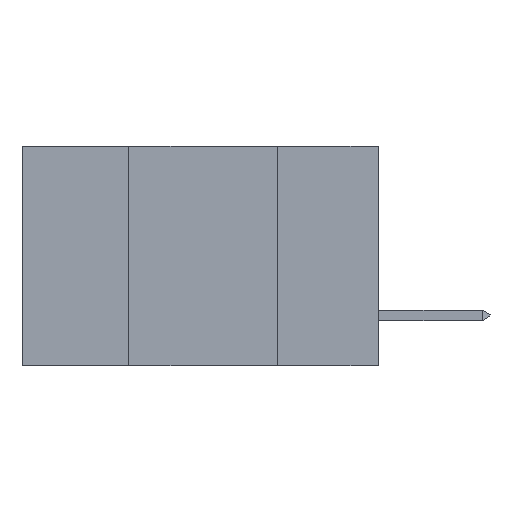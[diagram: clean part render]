
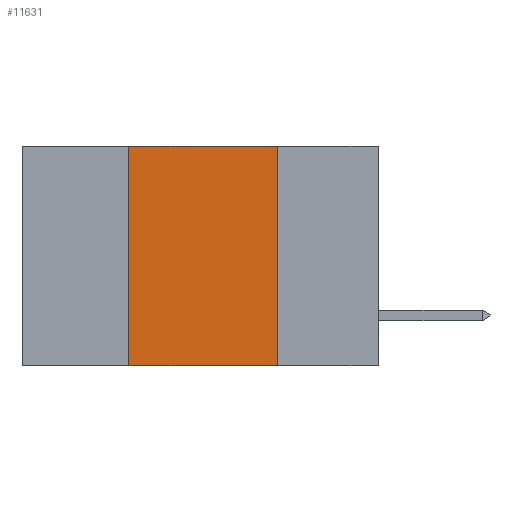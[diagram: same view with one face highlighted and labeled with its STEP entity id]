
A CAD part, left-side view. The second image highlights one B-rep face of the part: STEP entity #11631.
In plain terms, the highlighted planar face has unit normal (-1, 0, 0).
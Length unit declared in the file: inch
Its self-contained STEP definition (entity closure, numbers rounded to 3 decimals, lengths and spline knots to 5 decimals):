
#169 = DIRECTION ( 'NONE',  ( 0., -1., 0. ) ) ;
#295 = FACE_OUTER_BOUND ( 'NONE', #2165, .T. ) ;
#682 = CARTESIAN_POINT ( 'NONE',  ( 0., 0.17, -0.37 ) ) ;
#980 = LINE ( 'NONE', #7083, #4422 ) ;
#1053 = DIRECTION ( 'NONE',  ( 0., 0., -1. ) ) ;
#1113 = ORIENTED_EDGE ( 'NONE', *, *, #5870, .F. ) ;
#1149 = VERTEX_POINT ( 'NONE', #6041 ) ;
#1762 = EDGE_CURVE ( 'NONE', #8543, #9903, #980, .T. ) ;
#2165 = EDGE_LOOP ( 'NONE', ( #9676, #13576, #1113, #6295 ) ) ;
#2291 = LINE ( 'NONE', #9536, #14117 ) ;
#2891 = DIRECTION ( 'NONE',  ( 0., 0., -1. ) ) ;
#3404 = CARTESIAN_POINT ( 'NONE',  ( 0., 0.6, 0. ) ) ;
#3687 = DIRECTION ( 'NONE',  ( 0., -1., 0. ) ) ;
#4422 = VECTOR ( 'NONE', #169, 39.37008 ) ;
#5262 = CARTESIAN_POINT ( 'NONE',  ( 0., 0.42, -0.37 ) ) ;
#5268 = VERTEX_POINT ( 'NONE', #5733 ) ;
#5733 = CARTESIAN_POINT ( 'NONE',  ( 0., 0.42, 0. ) ) ;
#5734 = VECTOR ( 'NONE', #13889, 39.37008 ) ;
#5870 = EDGE_CURVE ( 'NONE', #8543, #5268, #11938, .T. ) ;
#6041 = CARTESIAN_POINT ( 'NONE',  ( 0., 0.17, 0. ) ) ;
#6295 = ORIENTED_EDGE ( 'NONE', *, *, #1762, .T. ) ;
#6999 = CARTESIAN_POINT ( 'NONE',  ( 0., 0.6, 0. ) ) ;
#7083 = CARTESIAN_POINT ( 'NONE',  ( 0., 0.6, -0.37 ) ) ;
#8543 = VERTEX_POINT ( 'NONE', #5262 ) ;
#8721 = AXIS2_PLACEMENT_3D ( 'NONE', #3404, #10389, #1053 ) ;
#8951 = VECTOR ( 'NONE', #3687, 39.37008 ) ;
#8956 = EDGE_CURVE ( 'NONE', #1149, #9903, #2291, .T. ) ;
#9357 = CARTESIAN_POINT ( 'NONE',  ( 0., 0.42, 0. ) ) ;
#9536 = CARTESIAN_POINT ( 'NONE',  ( 0., 0.17, 0. ) ) ;
#9676 = ORIENTED_EDGE ( 'NONE', *, *, #8956, .F. ) ;
#9903 = VERTEX_POINT ( 'NONE', #682 ) ;
#10246 = PLANE ( 'NONE',  #8721 ) ;
#10389 = DIRECTION ( 'NONE',  ( 1., 0., 0. ) ) ;
#11231 = EDGE_CURVE ( 'NONE', #5268, #1149, #12152, .T. ) ;
#11631 = ADVANCED_FACE ( 'NONE', ( #295 ), #10246, .F. ) ;
#11938 = LINE ( 'NONE', #9357, #5734 ) ;
#12152 = LINE ( 'NONE', #6999, #8951 ) ;
#13576 = ORIENTED_EDGE ( 'NONE', *, *, #11231, .F. ) ;
#13889 = DIRECTION ( 'NONE',  ( 0., 0., 1. ) ) ;
#14117 = VECTOR ( 'NONE', #2891, 39.37008 ) ;
